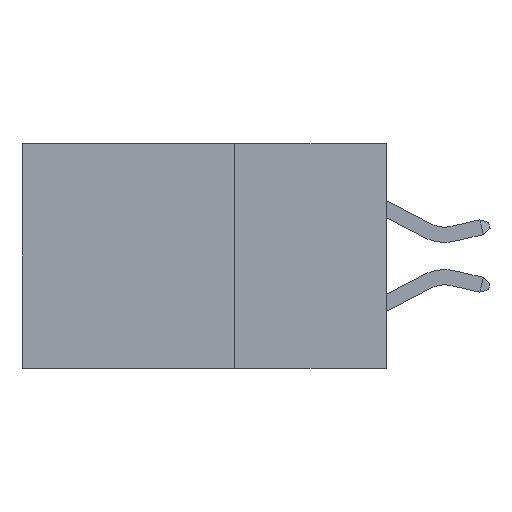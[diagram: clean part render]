
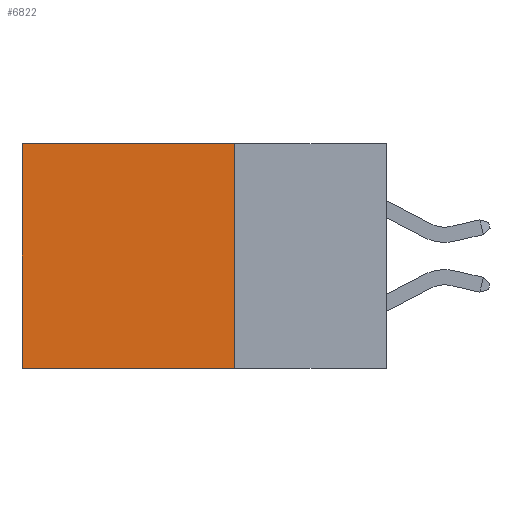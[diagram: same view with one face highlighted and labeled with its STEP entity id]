
A CAD part, left-side view. The second image highlights one B-rep face of the part: STEP entity #6822.
In plain terms, the highlighted planar face has unit normal (-1, 0, 0).
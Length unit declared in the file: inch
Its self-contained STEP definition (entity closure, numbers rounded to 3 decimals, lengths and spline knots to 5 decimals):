
#283 = DIRECTION ( 'NONE',  ( 0., 0., -1. ) ) ;
#721 = VECTOR ( 'NONE', #8503, 39.37008 ) ;
#912 = LINE ( 'NONE', #6324, #4984 ) ;
#998 = CARTESIAN_POINT ( 'NONE',  ( 0.298, 0.25, 0. ) ) ;
#1081 = CARTESIAN_POINT ( 'NONE',  ( 0.298, 0.25, -0.37 ) ) ;
#1497 = PLANE ( 'NONE',  #5256 ) ;
#2243 = EDGE_CURVE ( 'NONE', #5122, #9088, #912, .T. ) ;
#2284 = LINE ( 'NONE', #1081, #721 ) ;
#2460 = EDGE_LOOP ( 'NONE', ( #8414, #5006, #8598, #3115 ) ) ;
#3102 = DIRECTION ( 'NONE',  ( 0., 0., -1. ) ) ;
#3115 = ORIENTED_EDGE ( 'NONE', *, *, #3515, .T. ) ;
#3461 = VECTOR ( 'NONE', #5333, 39.37008 ) ;
#3515 = EDGE_CURVE ( 'NONE', #5122, #5811, #9220, .T. ) ;
#3552 = VERTEX_POINT ( 'NONE', #7257 ) ;
#3786 = VECTOR ( 'NONE', #283, 39.37008 ) ;
#4382 = CARTESIAN_POINT ( 'NONE',  ( 0.298, 0.6, 0. ) ) ;
#4984 = VECTOR ( 'NONE', #6285, 39.37008 ) ;
#5006 = ORIENTED_EDGE ( 'NONE', *, *, #6507, .F. ) ;
#5122 = VERTEX_POINT ( 'NONE', #5842 ) ;
#5256 = AXIS2_PLACEMENT_3D ( 'NONE', #6814, #7517, #3102 ) ;
#5333 = DIRECTION ( 'NONE',  ( 0., 1., 0. ) ) ;
#5533 = CARTESIAN_POINT ( 'NONE',  ( 0.298, 0.6, 0. ) ) ;
#5542 = EDGE_CURVE ( 'NONE', #5811, #3552, #5784, .T. ) ;
#5784 = LINE ( 'NONE', #5533, #3786 ) ;
#5811 = VERTEX_POINT ( 'NONE', #4382 ) ;
#5842 = CARTESIAN_POINT ( 'NONE',  ( 0.298, 0.25, 0. ) ) ;
#6285 = DIRECTION ( 'NONE',  ( 0., 0., -1. ) ) ;
#6324 = CARTESIAN_POINT ( 'NONE',  ( 0.298, 0.25, 0. ) ) ;
#6507 = EDGE_CURVE ( 'NONE', #9088, #3552, #2284, .T. ) ;
#6814 = CARTESIAN_POINT ( 'NONE',  ( 0.298, 0.25, 0. ) ) ;
#6822 = ADVANCED_FACE ( 'NONE', ( #9084 ), #1497, .F. ) ;
#7257 = CARTESIAN_POINT ( 'NONE',  ( 0.298, 0.6, -0.37 ) ) ;
#7517 = DIRECTION ( 'NONE',  ( 1., 0., 0. ) ) ;
#8414 = ORIENTED_EDGE ( 'NONE', *, *, #5542, .T. ) ;
#8503 = DIRECTION ( 'NONE',  ( 0., 1., 0. ) ) ;
#8598 = ORIENTED_EDGE ( 'NONE', *, *, #2243, .F. ) ;
#9084 = FACE_OUTER_BOUND ( 'NONE', #2460, .T. ) ;
#9088 = VERTEX_POINT ( 'NONE', #9173 ) ;
#9173 = CARTESIAN_POINT ( 'NONE',  ( 0.298, 0.25, -0.37 ) ) ;
#9220 = LINE ( 'NONE', #998, #3461 ) ;
